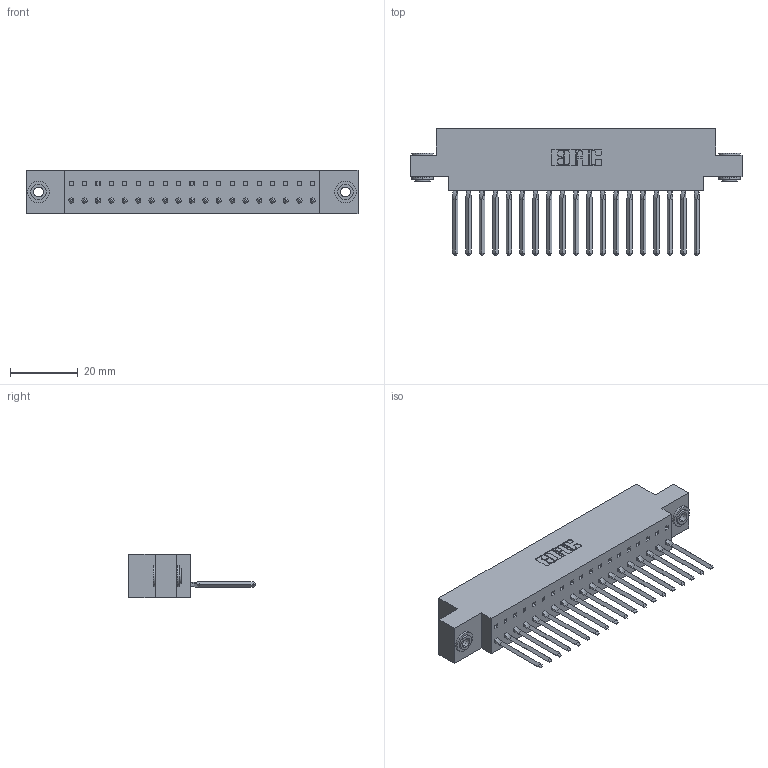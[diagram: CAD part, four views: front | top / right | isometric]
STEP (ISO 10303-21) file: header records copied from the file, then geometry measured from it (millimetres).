
FILE_DESCRIPTION (( 'STEP AP203' ), '1' );
FILE_NAME ('317-019-541-603.STEP', '2020-02-27T16:22:54', ( '' ), ( '' ), 'SwSTEP 2.0', 'SolidWorks 2016', '' );
FILE_SCHEMA (( 'CONFIG_CONTROL_DESIGN' ));
Length unit declared in the file: inch
Products named in the file (4): 317 Part_.156 Dia - TH; 317-290-002_541; 345-250-002_345-250-002-102; 317-019-541-603
Assembly tree (22 placements, depth 2):
  317-019-541-603
    317 Part_.156 Dia - TH
    317-290-002_541  x19
    345-250-002_345-250-002-102  x2
Bounding box: 97.99 x 37.34 x 12.7 mm (x, y, z)
Volume: 15203.4 mm3; surface area: 20931.3 mm2
Topology: 22 solids, 22 shells, 3028 faces, 8597 edges, 5588 vertices
Faces by surface type: plane 2424, cylinder 520, bspline 76, cone 8
Entity records: 32263 total; most frequent: CARTESIAN_POINT 6333, ORIENTED_EDGE 5598, DIRECTION 4623, EDGE_CURVE 2799, VECTOR 2411, LINE 2411, VERTEX_POINT 1856, AXIS2_PLACEMENT_3D 1106
